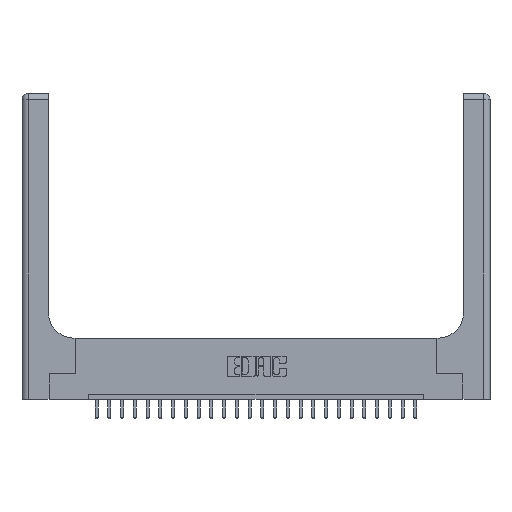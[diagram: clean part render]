
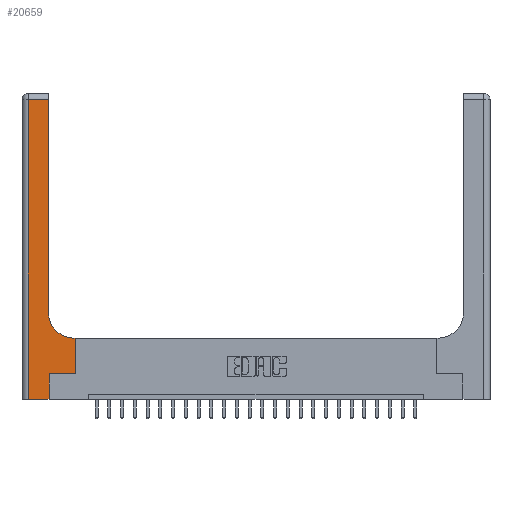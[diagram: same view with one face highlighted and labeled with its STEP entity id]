
A CAD part, top view. The second image highlights one B-rep face of the part: STEP entity #20659.
In plain terms, the highlighted planar face has unit normal (0, 0, 1).
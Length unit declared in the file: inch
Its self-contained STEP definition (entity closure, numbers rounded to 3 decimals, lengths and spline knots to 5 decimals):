
#717 = CARTESIAN_POINT ( 'NONE',  ( 0.26, 0.85, 0.37 ) ) ;
#719 = ORIENTED_EDGE ( 'NONE', *, *, #15554, .T. ) ;
#736 = CARTESIAN_POINT ( 'NONE',  ( 0.51, 0.85, 0.37 ) ) ;
#1460 = VECTOR ( 'NONE', #7829, 39.37008 ) ;
#1904 = CARTESIAN_POINT ( 'NONE',  ( 0.26, 2.94, 0.37 ) ) ;
#2017 = EDGE_CURVE ( 'NONE', #22028, #22830, #3205, .T. ) ;
#2435 = CARTESIAN_POINT ( 'NONE',  ( 0.528, 0.6, 0.37 ) ) ;
#2510 = ORIENTED_EDGE ( 'NONE', *, *, #14725, .T. ) ;
#2893 = FACE_OUTER_BOUND ( 'NONE', #11512, .T. ) ;
#3108 = ORIENTED_EDGE ( 'NONE', *, *, #3943, .T. ) ;
#3205 = CIRCLE ( 'NONE', #20262, 0.25 ) ;
#3939 = DIRECTION ( 'NONE',  ( 0., 1., 0. ) ) ;
#3943 = EDGE_CURVE ( 'NONE', #18775, #21994, #19667, .T. ) ;
#4090 = CARTESIAN_POINT ( 'NONE',  ( 0.265, 0., 0.37 ) ) ;
#4157 = DIRECTION ( 'NONE',  ( 1., 0., 0. ) ) ;
#4367 = DIRECTION ( 'NONE',  ( 0., -1., 0. ) ) ;
#4490 = ORIENTED_EDGE ( 'NONE', *, *, #20499, .T. ) ;
#4777 = ORIENTED_EDGE ( 'NONE', *, *, #15343, .T. ) ;
#4888 = CARTESIAN_POINT ( 'NONE',  ( 0.06, 3., 0.37 ) ) ;
#5993 = VERTEX_POINT ( 'NONE', #17562 ) ;
#6365 = ORIENTED_EDGE ( 'NONE', *, *, #11310, .T. ) ;
#7138 = CARTESIAN_POINT ( 'NONE',  ( 0.26, 0.6, 0.37 ) ) ;
#7829 = DIRECTION ( 'NONE',  ( 1., 0., 0. ) ) ;
#8151 = CARTESIAN_POINT ( 'NONE',  ( 0., 3., 0.37 ) ) ;
#8507 = CARTESIAN_POINT ( 'NONE',  ( 0., 0., 0.37 ) ) ;
#10125 = DIRECTION ( 'NONE',  ( 0., 0., -1. ) ) ;
#10314 = DIRECTION ( 'NONE',  ( 1., 0., 0. ) ) ;
#10538 = CARTESIAN_POINT ( 'NONE',  ( 0.265, 0.25, 0.37 ) ) ;
#10772 = CARTESIAN_POINT ( 'NONE',  ( 0.51, 0.6, 0.37 ) ) ;
#10889 = CARTESIAN_POINT ( 'NONE',  ( 0.265, 0., 0.37 ) ) ;
#11310 = EDGE_CURVE ( 'NONE', #5993, #13126, #11572, .T. ) ;
#11512 = EDGE_LOOP ( 'NONE', ( #15499, #4490, #3108, #4777, #21884, #2510, #6365, #719, #13573 ) ) ;
#11572 = LINE ( 'NONE', #11767, #14425 ) ;
#11730 = VECTOR ( 'NONE', #18860, 39.37008 ) ;
#11767 = CARTESIAN_POINT ( 'NONE',  ( 0.528, 0.25, 0.37 ) ) ;
#12118 = LINE ( 'NONE', #21131, #16730 ) ;
#12480 = VECTOR ( 'NONE', #3939, 39.37008 ) ;
#12681 = VERTEX_POINT ( 'NONE', #10538 ) ;
#12688 = CARTESIAN_POINT ( 'NONE',  ( 0.06, 0., 0.37 ) ) ;
#13126 = VERTEX_POINT ( 'NONE', #2435 ) ;
#13470 = PLANE ( 'NONE',  #18514 ) ;
#13573 = ORIENTED_EDGE ( 'NONE', *, *, #2017, .T. ) ;
#14425 = VECTOR ( 'NONE', #19132, 39.37008 ) ;
#14725 = EDGE_CURVE ( 'NONE', #12681, #5993, #22544, .T. ) ;
#15311 = DIRECTION ( 'NONE',  ( 0., 0., -1. ) ) ;
#15343 = EDGE_CURVE ( 'NONE', #21994, #17593, #18822, .T. ) ;
#15499 = ORIENTED_EDGE ( 'NONE', *, *, #18570, .T. ) ;
#15554 = EDGE_CURVE ( 'NONE', #13126, #22028, #23361, .T. ) ;
#16268 = VECTOR ( 'NONE', #10314, 39.37008 ) ;
#16632 = LINE ( 'NONE', #20520, #11730 ) ;
#16730 = VECTOR ( 'NONE', #21048, 39.37008 ) ;
#16739 = EDGE_CURVE ( 'NONE', #17593, #12681, #20460, .T. ) ;
#17398 = VECTOR ( 'NONE', #4367, 39.37008 ) ;
#17562 = CARTESIAN_POINT ( 'NONE',  ( 0.528, 0.25, 0.37 ) ) ;
#17593 = VERTEX_POINT ( 'NONE', #10889 ) ;
#18514 = AXIS2_PLACEMENT_3D ( 'NONE', #8151, #10125, #22888 ) ;
#18570 = EDGE_CURVE ( 'NONE', #22830, #21670, #12118, .T. ) ;
#18775 = VERTEX_POINT ( 'NONE', #21441 ) ;
#18822 = LINE ( 'NONE', #8507, #16268 ) ;
#18860 = DIRECTION ( 'NONE',  ( -1., 0., 0. ) ) ;
#19132 = DIRECTION ( 'NONE',  ( 0., 1., 0. ) ) ;
#19667 = LINE ( 'NONE', #4888, #17398 ) ;
#19883 = DIRECTION ( 'NONE',  ( -1., 0., 0. ) ) ;
#20229 = VECTOR ( 'NONE', #19883, 39.37008 ) ;
#20262 = AXIS2_PLACEMENT_3D ( 'NONE', #736, #15311, #4157 ) ;
#20460 = LINE ( 'NONE', #4090, #12480 ) ;
#20499 = EDGE_CURVE ( 'NONE', #21670, #18775, #16632, .T. ) ;
#20520 = CARTESIAN_POINT ( 'NONE',  ( 0., 2.94, 0.37 ) ) ;
#20590 = CARTESIAN_POINT ( 'NONE',  ( 0.265, 0.25, 0.37 ) ) ;
#20659 = ADVANCED_FACE ( 'NONE', ( #2893 ), #13470, .F. ) ;
#21048 = DIRECTION ( 'NONE',  ( 0., 1., 0. ) ) ;
#21131 = CARTESIAN_POINT ( 'NONE',  ( 0.26, 3., 0.37 ) ) ;
#21441 = CARTESIAN_POINT ( 'NONE',  ( 0.06, 2.94, 0.37 ) ) ;
#21670 = VERTEX_POINT ( 'NONE', #1904 ) ;
#21884 = ORIENTED_EDGE ( 'NONE', *, *, #16739, .T. ) ;
#21994 = VERTEX_POINT ( 'NONE', #12688 ) ;
#22028 = VERTEX_POINT ( 'NONE', #10772 ) ;
#22544 = LINE ( 'NONE', #20590, #1460 ) ;
#22830 = VERTEX_POINT ( 'NONE', #717 ) ;
#22888 = DIRECTION ( 'NONE',  ( -1., 0., 0. ) ) ;
#23361 = LINE ( 'NONE', #7138, #20229 ) ;
